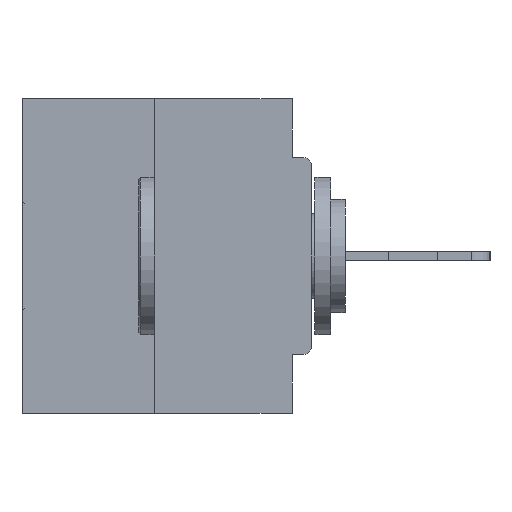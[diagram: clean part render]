
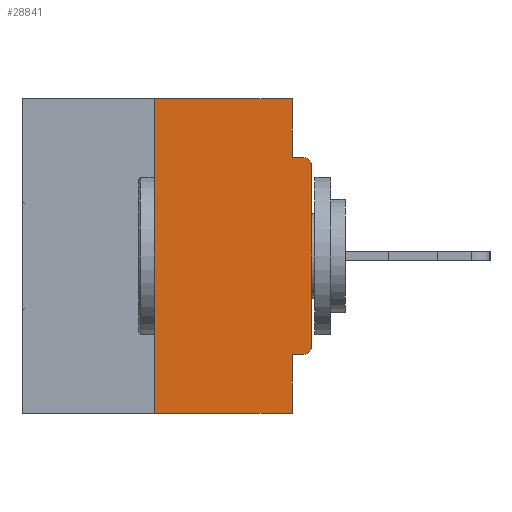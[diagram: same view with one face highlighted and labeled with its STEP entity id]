
A CAD part, left-side view. The second image highlights one B-rep face of the part: STEP entity #28841.
In plain terms, the highlighted planar face has unit normal (-1, 0, 0).
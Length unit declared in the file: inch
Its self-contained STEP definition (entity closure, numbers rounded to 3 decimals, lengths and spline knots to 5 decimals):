
#312 = VECTOR ( 'NONE', #27256, 39.37008 ) ;
#1000 = ORIENTED_EDGE ( 'NONE', *, *, #5381, .F. ) ;
#1075 = DIRECTION ( 'NONE',  ( 0., 1., 0. ) ) ;
#1837 = ORIENTED_EDGE ( 'NONE', *, *, #2527, .T. ) ;
#2221 = DIRECTION ( 'NONE',  ( 0., -1., 0. ) ) ;
#2514 = CARTESIAN_POINT ( 'NONE',  ( 0., 0.031, -0.5 ) ) ;
#2527 = EDGE_CURVE ( 'NONE', #25995, #27734, #13971, .T. ) ;
#2617 = DIRECTION ( 'NONE',  ( 0., 0., -1. ) ) ;
#3635 = LINE ( 'NONE', #14876, #5129 ) ;
#4001 = CARTESIAN_POINT ( 'NONE',  ( 0., 0.031, -0.0935 ) ) ;
#4274 = VECTOR ( 'NONE', #30136, 39.37008 ) ;
#4656 = EDGE_CURVE ( 'NONE', #14630, #16620, #22185, .T. ) ;
#4753 = VERTEX_POINT ( 'NONE', #32060 ) ;
#5129 = VECTOR ( 'NONE', #1075, 39.37008 ) ;
#5205 = DIRECTION ( 'NONE',  ( 1., 0., 0. ) ) ;
#5381 = EDGE_CURVE ( 'NONE', #23661, #6643, #27579, .T. ) ;
#5611 = ORIENTED_EDGE ( 'NONE', *, *, #29052, .T. ) ;
#6466 = DIRECTION ( 'NONE',  ( 0., 0., -1. ) ) ;
#6643 = VERTEX_POINT ( 'NONE', #36171 ) ;
#6697 = ORIENTED_EDGE ( 'NONE', *, *, #19925, .T. ) ;
#7267 = VECTOR ( 'NONE', #18534, 39.37008 ) ;
#7766 = VECTOR ( 'NONE', #14238, 39.37008 ) ;
#8243 = LINE ( 'NONE', #33489, #13755 ) ;
#8872 = VECTOR ( 'NONE', #25015, 39.37008 ) ;
#8931 = VECTOR ( 'NONE', #2221, 39.37008 ) ;
#9049 = DIRECTION ( 'NONE',  ( -1., 0., 0. ) ) ;
#9410 = VERTEX_POINT ( 'NONE', #12782 ) ;
#10401 = ORIENTED_EDGE ( 'NONE', *, *, #4656, .F. ) ;
#10588 = EDGE_CURVE ( 'NONE', #32871, #28926, #35533, .T. ) ;
#10809 = CARTESIAN_POINT ( 'NONE',  ( 0., 0.25, 0. ) ) ;
#11032 = CARTESIAN_POINT ( 'NONE',  ( 0., 0.46, 0. ) ) ;
#11120 = CARTESIAN_POINT ( 'NONE',  ( 0., 0.031, -0.5 ) ) ;
#11328 = ORIENTED_EDGE ( 'NONE', *, *, #26238, .F. ) ;
#11470 = CARTESIAN_POINT ( 'NONE',  ( 0., 0., -0.3915 ) ) ;
#12782 = CARTESIAN_POINT ( 'NONE',  ( 0., 0.015, -0.4065 ) ) ;
#13088 = CARTESIAN_POINT ( 'NONE',  ( 0., 0., -0.0935 ) ) ;
#13606 = DIRECTION ( 'NONE',  ( 0., 0., -1. ) ) ;
#13755 = VECTOR ( 'NONE', #13606, 39.37008 ) ;
#13971 = LINE ( 'NONE', #31264, #8872 ) ;
#14203 = FACE_OUTER_BOUND ( 'NONE', #15146, .T. ) ;
#14238 = DIRECTION ( 'NONE',  ( 0., 0., -1. ) ) ;
#14630 = VERTEX_POINT ( 'NONE', #25403 ) ;
#14876 = CARTESIAN_POINT ( 'NONE',  ( 0., 0., -0.4065 ) ) ;
#15125 = CARTESIAN_POINT ( 'NONE',  ( 0., 0., -0.1085 ) ) ;
#15146 = EDGE_LOOP ( 'NONE', ( #11328, #1000, #26420, #10401, #24011, #5611, #1837, #6697, #18599, #21796 ) ) ;
#15461 = DIRECTION ( 'NONE',  ( -1., 0., 0. ) ) ;
#16620 = VERTEX_POINT ( 'NONE', #2514 ) ;
#18534 = DIRECTION ( 'NONE',  ( 0., -1., 0. ) ) ;
#18599 = ORIENTED_EDGE ( 'NONE', *, *, #10588, .F. ) ;
#19085 = CARTESIAN_POINT ( 'NONE',  ( 0., 0.015, -0.1085 ) ) ;
#19925 = EDGE_CURVE ( 'NONE', #27734, #28926, #22982, .T. ) ;
#20573 = LINE ( 'NONE', #26999, #7267 ) ;
#21796 = ORIENTED_EDGE ( 'NONE', *, *, #32613, .F. ) ;
#21885 = AXIS2_PLACEMENT_3D ( 'NONE', #25804, #9049, #6466 ) ;
#22185 = LINE ( 'NONE', #11120, #7766 ) ;
#22217 = DIRECTION ( 'NONE',  ( 0., 0., -1. ) ) ;
#22867 = CARTESIAN_POINT ( 'NONE',  ( 0., 0.46, 0. ) ) ;
#22982 = CIRCLE ( 'NONE', #29475, 0.015 ) ;
#23240 = CARTESIAN_POINT ( 'NONE',  ( 0., 0.015, -0.0935 ) ) ;
#23661 = VERTEX_POINT ( 'NONE', #35165 ) ;
#24011 = ORIENTED_EDGE ( 'NONE', *, *, #35662, .F. ) ;
#24535 = EDGE_CURVE ( 'NONE', #23661, #16620, #20573, .T. ) ;
#25015 = DIRECTION ( 'NONE',  ( 0., 0., 1. ) ) ;
#25403 = CARTESIAN_POINT ( 'NONE',  ( 0., 0.031, -0.4065 ) ) ;
#25804 = CARTESIAN_POINT ( 'NONE',  ( 0., 0.015, -0.3915 ) ) ;
#25995 = VERTEX_POINT ( 'NONE', #11470 ) ;
#26238 = EDGE_CURVE ( 'NONE', #6643, #4753, #36250, .T. ) ;
#26420 = ORIENTED_EDGE ( 'NONE', *, *, #24535, .T. ) ;
#26999 = CARTESIAN_POINT ( 'NONE',  ( 0., 0.46, -0.5 ) ) ;
#27167 = CIRCLE ( 'NONE', #21885, 0.015 ) ;
#27256 = DIRECTION ( 'NONE',  ( 0., -1., 0. ) ) ;
#27579 = LINE ( 'NONE', #10809, #4274 ) ;
#27734 = VERTEX_POINT ( 'NONE', #15125 ) ;
#28841 = ADVANCED_FACE ( 'NONE', ( #14203 ), #36297, .F. ) ;
#28926 = VERTEX_POINT ( 'NONE', #23240 ) ;
#29052 = EDGE_CURVE ( 'NONE', #9410, #25995, #27167, .T. ) ;
#29475 = AXIS2_PLACEMENT_3D ( 'NONE', #19085, #15461, #22217 ) ;
#29504 = AXIS2_PLACEMENT_3D ( 'NONE', #22867, #5205, #2617 ) ;
#30136 = DIRECTION ( 'NONE',  ( 0., 0., 1. ) ) ;
#31264 = CARTESIAN_POINT ( 'NONE',  ( 0., 0., 0. ) ) ;
#32060 = CARTESIAN_POINT ( 'NONE',  ( 0., 0.031, 0. ) ) ;
#32613 = EDGE_CURVE ( 'NONE', #4753, #32871, #8243, .T. ) ;
#32871 = VERTEX_POINT ( 'NONE', #4001 ) ;
#33489 = CARTESIAN_POINT ( 'NONE',  ( 0., 0.031, 0. ) ) ;
#35165 = CARTESIAN_POINT ( 'NONE',  ( 0., 0.25, -0.5 ) ) ;
#35533 = LINE ( 'NONE', #13088, #8931 ) ;
#35662 = EDGE_CURVE ( 'NONE', #9410, #14630, #3635, .T. ) ;
#36171 = CARTESIAN_POINT ( 'NONE',  ( 0., 0.25, 0. ) ) ;
#36250 = LINE ( 'NONE', #11032, #312 ) ;
#36297 = PLANE ( 'NONE',  #29504 ) ;
